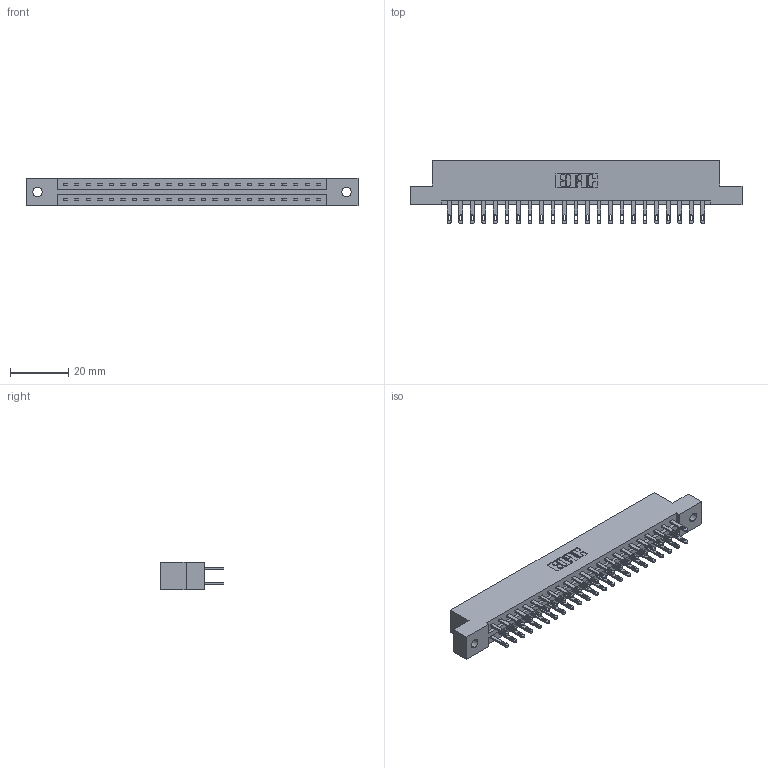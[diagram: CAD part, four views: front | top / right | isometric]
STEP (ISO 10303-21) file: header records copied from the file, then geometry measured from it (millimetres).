
FILE_DESCRIPTION (( 'STEP AP203' ), '1' );
FILE_NAME ('887-046-500-202.STEP', '2020-09-21T00:38:28', ( '' ), ( '' ), 'SwSTEP 2.0', 'SolidWorks 2020', '' );
FILE_SCHEMA (( 'CONFIG_CONTROL_DESIGN' ));
Length unit declared in the file: inch
Products named in the file (3): 837 Part_Flush Mounting Lugs - 0.128 Dia; 345-292-001_345-293-100; 887-046-500-202
Assembly tree (47 placements, depth 2):
  887-046-500-202
    837 Part_Flush Mounting Lugs - 0.128 Dia
    345-292-001_345-293-100  x46
Bounding box: 114.15 x 21.85 x 9.4 mm (x, y, z)
Volume: 11880.8 mm3; surface area: 13484.3 mm2
Topology: 47 solids, 47 shells, 2414 faces, 7349 edges, 4898 vertices
Faces by surface type: plane 1542, cylinder 872
Entity records: 20223 total; most frequent: CARTESIAN_POINT 3422, ORIENTED_EDGE 3358, DIRECTION 2947, EDGE_CURVE 1679, LINE 1547, VECTOR 1547, VERTEX_POINT 1118, AXIS2_PLACEMENT_3D 700
